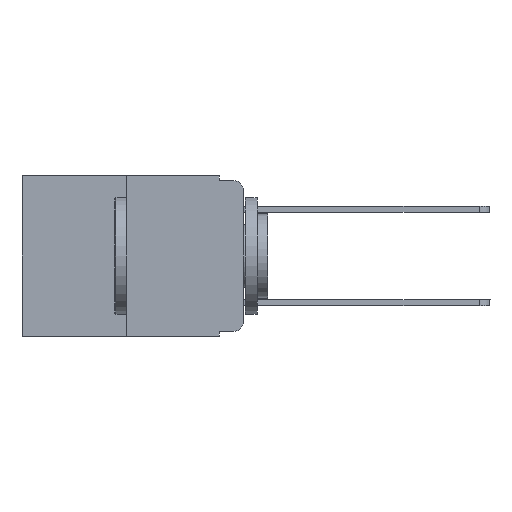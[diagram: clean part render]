
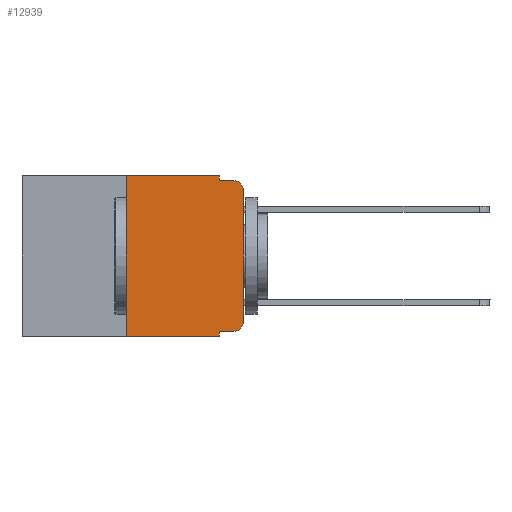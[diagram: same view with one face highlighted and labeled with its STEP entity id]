
A CAD part, left-side view. The second image highlights one B-rep face of the part: STEP entity #12939.
In plain terms, the highlighted planar face has unit normal (-1, 0, 0).
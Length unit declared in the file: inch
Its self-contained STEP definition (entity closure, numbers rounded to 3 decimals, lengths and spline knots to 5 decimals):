
#15 = CARTESIAN_POINT ( 'NONE',  ( 0., 0.051, -0.01 ) ) ;
#327 = DIRECTION ( 'NONE',  ( 0., 0., 1. ) ) ;
#331 = CIRCLE ( 'NONE', #6619, 0.02 ) ;
#788 = VECTOR ( 'NONE', #9808, 39.37008 ) ;
#832 = VECTOR ( 'NONE', #7250, 39.37008 ) ;
#1376 = EDGE_CURVE ( 'NONE', #13539, #14494, #16395, .T. ) ;
#1513 = VERTEX_POINT ( 'NONE', #14163 ) ;
#1861 = CARTESIAN_POINT ( 'NONE',  ( 0., 0.02, -0.01 ) ) ;
#2114 = EDGE_CURVE ( 'NONE', #6430, #6993, #14919, .T. ) ;
#2411 = LINE ( 'NONE', #5681, #6304 ) ;
#2600 = EDGE_CURVE ( 'NONE', #15158, #10678, #2411, .T. ) ;
#2694 = DIRECTION ( 'NONE',  ( -1., 0., 0. ) ) ;
#2779 = ORIENTED_EDGE ( 'NONE', *, *, #4020, .T. ) ;
#2854 = ORIENTED_EDGE ( 'NONE', *, *, #1376, .F. ) ;
#2864 = CARTESIAN_POINT ( 'NONE',  ( 0., 0.473, 0. ) ) ;
#3184 = FACE_OUTER_BOUND ( 'NONE', #11012, .T. ) ;
#3274 = EDGE_CURVE ( 'NONE', #1513, #13539, #4241, .T. ) ;
#3284 = ORIENTED_EDGE ( 'NONE', *, *, #7729, .F. ) ;
#3570 = ORIENTED_EDGE ( 'NONE', *, *, #7096, .F. ) ;
#3723 = LINE ( 'NONE', #7164, #7003 ) ;
#3835 = ORIENTED_EDGE ( 'NONE', *, *, #2114, .T. ) ;
#3895 = CARTESIAN_POINT ( 'NONE',  ( 0., 0.02, -0.03 ) ) ;
#4013 = DIRECTION ( 'NONE',  ( 0., -1., 0. ) ) ;
#4020 = EDGE_CURVE ( 'NONE', #4043, #6466, #13815, .T. ) ;
#4043 = VERTEX_POINT ( 'NONE', #16913 ) ;
#4241 = LINE ( 'NONE', #5950, #788 ) ;
#4366 = ORIENTED_EDGE ( 'NONE', *, *, #16728, .F. ) ;
#5006 = PLANE ( 'NONE',  #9780 ) ;
#5543 = CARTESIAN_POINT ( 'NONE',  ( 0., 0.25, 0. ) ) ;
#5639 = DIRECTION ( 'NONE',  ( 0., 0., -1. ) ) ;
#5681 = CARTESIAN_POINT ( 'NONE',  ( 0., 0.051, -0.333 ) ) ;
#5950 = CARTESIAN_POINT ( 'NONE',  ( 0., 0.051, 0. ) ) ;
#6111 = CIRCLE ( 'NONE', #16034, 0.02 ) ;
#6304 = VECTOR ( 'NONE', #9442, 39.37008 ) ;
#6430 = VERTEX_POINT ( 'NONE', #14481 ) ;
#6466 = VERTEX_POINT ( 'NONE', #14361 ) ;
#6619 = AXIS2_PLACEMENT_3D ( 'NONE', #3895, #2694, #10516 ) ;
#6993 = VERTEX_POINT ( 'NONE', #10717 ) ;
#7003 = VECTOR ( 'NONE', #15133, 39.37008 ) ;
#7096 = EDGE_CURVE ( 'NONE', #6430, #15481, #14766, .T. ) ;
#7112 = ORIENTED_EDGE ( 'NONE', *, *, #3274, .F. ) ;
#7164 = CARTESIAN_POINT ( 'NONE',  ( 0., 0.051, 0. ) ) ;
#7250 = DIRECTION ( 'NONE',  ( 0., -1., 0. ) ) ;
#7313 = ORIENTED_EDGE ( 'NONE', *, *, #2600, .T. ) ;
#7505 = ORIENTED_EDGE ( 'NONE', *, *, #14864, .T. ) ;
#7608 = CARTESIAN_POINT ( 'NONE',  ( 0., 0.473, 0. ) ) ;
#7685 = VECTOR ( 'NONE', #15252, 39.37008 ) ;
#7729 = EDGE_CURVE ( 'NONE', #15481, #1513, #15033, .T. ) ;
#7779 = DIRECTION ( 'NONE',  ( 1., 0., 0. ) ) ;
#8136 = CARTESIAN_POINT ( 'NONE',  ( 0., 0.02, -0.313 ) ) ;
#8405 = CARTESIAN_POINT ( 'NONE',  ( 0., 0.051, -0.333 ) ) ;
#8464 = VECTOR ( 'NONE', #4013, 39.37008 ) ;
#8744 = CARTESIAN_POINT ( 'NONE',  ( 0., 0.473, -0.343 ) ) ;
#8980 = DIRECTION ( 'NONE',  ( 0., 0., -1. ) ) ;
#9442 = DIRECTION ( 'NONE',  ( 0., -1., 0. ) ) ;
#9780 = AXIS2_PLACEMENT_3D ( 'NONE', #7608, #7779, #8980 ) ;
#9808 = DIRECTION ( 'NONE',  ( 0., 0., -1. ) ) ;
#10252 = VECTOR ( 'NONE', #327, 39.37008 ) ;
#10516 = DIRECTION ( 'NONE',  ( 0., 0., -1. ) ) ;
#10678 = VERTEX_POINT ( 'NONE', #16211 ) ;
#10717 = CARTESIAN_POINT ( 'NONE',  ( 0., 0.051, -0.343 ) ) ;
#11012 = EDGE_LOOP ( 'NONE', ( #2779, #7505, #2854, #7112, #3284, #3570, #3835, #4366, #7313, #13281 ) ) ;
#11272 = DIRECTION ( 'NONE',  ( 0., -1., 0. ) ) ;
#11414 = VECTOR ( 'NONE', #11272, 39.37008 ) ;
#11869 = EDGE_CURVE ( 'NONE', #10678, #4043, #6111, .T. ) ;
#12939 = ADVANCED_FACE ( 'NONE', ( #3184 ), #5006, .F. ) ;
#13281 = ORIENTED_EDGE ( 'NONE', *, *, #11869, .T. ) ;
#13375 = DIRECTION ( 'NONE',  ( -1., 0., 0. ) ) ;
#13539 = VERTEX_POINT ( 'NONE', #15 ) ;
#13815 = LINE ( 'NONE', #14079, #7685 ) ;
#14079 = CARTESIAN_POINT ( 'NONE',  ( 0., 0., 0. ) ) ;
#14163 = CARTESIAN_POINT ( 'NONE',  ( 0., 0.051, 0. ) ) ;
#14361 = CARTESIAN_POINT ( 'NONE',  ( 0., 0., -0.03 ) ) ;
#14481 = CARTESIAN_POINT ( 'NONE',  ( 0., 0.25, -0.343 ) ) ;
#14494 = VERTEX_POINT ( 'NONE', #1861 ) ;
#14766 = LINE ( 'NONE', #5543, #10252 ) ;
#14864 = EDGE_CURVE ( 'NONE', #6466, #14494, #331, .T. ) ;
#14919 = LINE ( 'NONE', #8744, #11414 ) ;
#14989 = CARTESIAN_POINT ( 'NONE',  ( 0., 0.051, -0.01 ) ) ;
#15033 = LINE ( 'NONE', #2864, #8464 ) ;
#15133 = DIRECTION ( 'NONE',  ( 0., 0., -1. ) ) ;
#15158 = VERTEX_POINT ( 'NONE', #8405 ) ;
#15252 = DIRECTION ( 'NONE',  ( 0., 0., 1. ) ) ;
#15481 = VERTEX_POINT ( 'NONE', #16836 ) ;
#16034 = AXIS2_PLACEMENT_3D ( 'NONE', #8136, #13375, #5639 ) ;
#16211 = CARTESIAN_POINT ( 'NONE',  ( 0., 0.02, -0.333 ) ) ;
#16395 = LINE ( 'NONE', #14989, #832 ) ;
#16728 = EDGE_CURVE ( 'NONE', #15158, #6993, #3723, .T. ) ;
#16836 = CARTESIAN_POINT ( 'NONE',  ( 0., 0.25, 0. ) ) ;
#16913 = CARTESIAN_POINT ( 'NONE',  ( 0., 0., -0.313 ) ) ;
